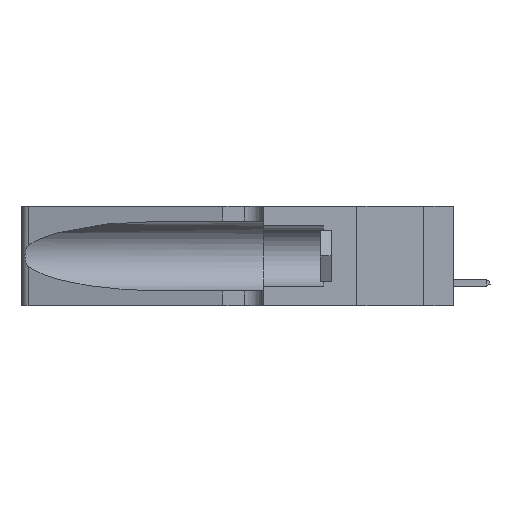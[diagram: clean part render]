
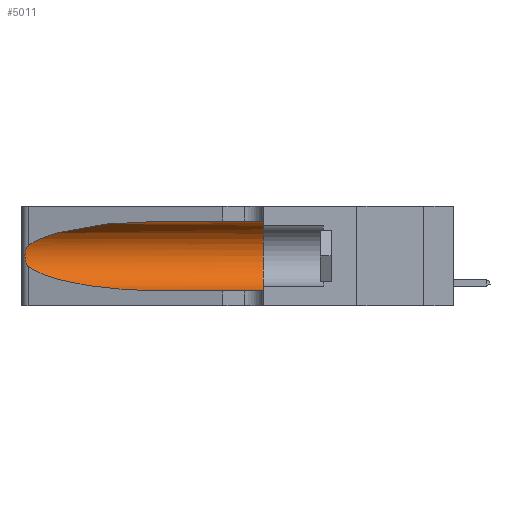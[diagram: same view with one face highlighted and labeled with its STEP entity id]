
A CAD part, left-side view. The second image highlights one B-rep face of the part: STEP entity #5011.
In plain terms, the highlighted cylindrical face has radius 3.308 mm (diameter 6.617 mm), a partial arc.
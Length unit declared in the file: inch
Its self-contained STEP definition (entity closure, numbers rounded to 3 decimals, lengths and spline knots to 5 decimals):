
#193 = EDGE_CURVE ( 'NONE', #3831, #10696, #7892, .T. ) ;
#352 = CARTESIAN_POINT ( 'NONE',  ( 0.1305, 0.35, 0.05475 ) ) ;
#851 = DIRECTION ( 'NONE',  ( 0., -1., 0. ) ) ;
#1454 = ORIENTED_EDGE ( 'NONE', *, *, #193, .T. ) ;
#1737 = CARTESIAN_POINT ( 'NONE',  ( 0.25854, 1.2359, 0.20912 ) ) ;
#1858 = CARTESIAN_POINT ( 'NONE',  ( 0.25487, 1.22718, 0.22369 ) ) ;
#1921 = CARTESIAN_POINT ( 'NONE',  ( 0.25789, 1.23486, 0.15765 ) ) ;
#2220 = CARTESIAN_POINT ( 'NONE',  ( 0.1305, 1.61858, 0.31525 ) ) ;
#2364 = EDGE_CURVE ( 'NONE', #7853, #3831, #17258, .T. ) ;
#3065 = ORIENTED_EDGE ( 'NONE', *, *, #10137, .T. ) ;
#3291 = CARTESIAN_POINT ( 'NONE',  ( 0.25639, 1.23186, 0.15144 ) ) ;
#3459 = LINE ( 'NONE', #2220, #13049 ) ;
#3567 = AXIS2_PLACEMENT_3D ( 'NONE', #7387, #4279, #14512 ) ;
#3663 = VECTOR ( 'NONE', #11412, 39.37008 ) ;
#3831 = VERTEX_POINT ( 'NONE', #13949 ) ;
#4229 = ORIENTED_EDGE ( 'NONE', *, *, #9082, .F. ) ;
#4279 = DIRECTION ( 'NONE',  ( 0., 1., 0. ) ) ;
#4333 = CYLINDRICAL_SURFACE ( 'NONE', #6088, 0.13025 ) ;
#4395 = CARTESIAN_POINT ( 'NONE',  ( 0.25555, 1.22994, 0.2215 ) ) ;
#4707 = CARTESIAN_POINT ( 'NONE',  ( 0.26017, 1.23833, 0.17102 ) ) ;
#4766 =( BOUNDED_CURVE ( )  B_SPLINE_CURVE ( 3, ( #9115, #17762, #9359, #6259 ),
 .UNSPECIFIED., .F., .T. ) 
 B_SPLINE_CURVE_WITH_KNOTS ( ( 4, 4 ),
 ( 1.5708, 2.84003 ),
 .UNSPECIFIED. ) 
 CURVE ( )  GEOMETRIC_REPRESENTATION_ITEM ( )  RATIONAL_B_SPLINE_CURVE ( ( 1., 0.87, 0.87, 1. ) ) 
 REPRESENTATION_ITEM ( '' )  );
#4895 = CARTESIAN_POINT ( 'NONE',  ( 0.25487, 1.22718, 0.14631 ) ) ;
#4959 = CARTESIAN_POINT ( 'NONE',  ( 0.26075, 1.23896, 0.19203 ) ) ;
#5011 = ADVANCED_FACE ( 'NONE', ( #8567 ), #4333, .F. ) ;
#5245 = VERTEX_POINT ( 'NONE', #8311 ) ;
#5905 = CARTESIAN_POINT ( 'NONE',  ( 0.25639, 1.23184, 0.21858 ) ) ;
#5938 = ORIENTED_EDGE ( 'NONE', *, *, #9003, .T. ) ;
#6088 = AXIS2_PLACEMENT_3D ( 'NONE', #13794, #12398, #15220 ) ;
#6259 = CARTESIAN_POINT ( 'NONE',  ( 0.25487, 1.22718, 0.22369 ) ) ;
#6638 = VERTEX_POINT ( 'NONE', #14657 ) ;
#7343 = CARTESIAN_POINT ( 'NONE',  ( 0.2373, 1.15595, 0.08982 ) ) ;
#7387 = CARTESIAN_POINT ( 'NONE',  ( 0.1305, 0.35, 0.185 ) ) ;
#7408 = CARTESIAN_POINT ( 'NONE',  ( 0.25487, 1.22718, 0.14631 ) ) ;
#7422 = CARTESIAN_POINT ( 'NONE',  ( 0.1305, 1.61858, 0.05475 ) ) ;
#7614 = CARTESIAN_POINT ( 'NONE',  ( 0.1305, 0.72297, 0.31525 ) ) ;
#7755 = CARTESIAN_POINT ( 'NONE',  ( 0.25555, 1.22993, 0.14849 ) ) ;
#7853 = VERTEX_POINT ( 'NONE', #14208 ) ;
#7892 = LINE ( 'NONE', #7422, #3663 ) ;
#8311 = CARTESIAN_POINT ( 'NONE',  ( 0.25487, 1.22718, 0.22369 ) ) ;
#8567 = FACE_OUTER_BOUND ( 'NONE', #14930, .T. ) ;
#9003 = EDGE_CURVE ( 'NONE', #16059, #5245, #4766, .T. ) ;
#9082 = EDGE_CURVE ( 'NONE', #6638, #10696, #15347, .T. ) ;
#9115 = CARTESIAN_POINT ( 'NONE',  ( 0.1305, 0.72297, 0.31525 ) ) ;
#9359 = CARTESIAN_POINT ( 'NONE',  ( 0.2373, 1.15595, 0.28018 ) ) ;
#10137 = EDGE_CURVE ( 'NONE', #5245, #7853, #15057, .T. ) ;
#10235 = CARTESIAN_POINT ( 'NONE',  ( 0.25787, 1.23484, 0.2124 ) ) ;
#10696 = VERTEX_POINT ( 'NONE', #352 ) ;
#11412 = DIRECTION ( 'NONE',  ( 0., -1., 0. ) ) ;
#11692 = CARTESIAN_POINT ( 'NONE',  ( 0.26018, 1.23835, 0.19895 ) ) ;
#11858 = EDGE_CURVE ( 'NONE', #16059, #6638, #3459, .T. ) ;
#11880 = CARTESIAN_POINT ( 'NONE',  ( 0.26075, 1.23896, 0.178 ) ) ;
#12398 = DIRECTION ( 'NONE',  ( 0., -1., 0. ) ) ;
#13049 = VECTOR ( 'NONE', #851, 39.37008 ) ;
#13094 = CARTESIAN_POINT ( 'NONE',  ( 0.1305, 0.72297, 0.05475 ) ) ;
#13436 = CARTESIAN_POINT ( 'NONE',  ( 0.25856, 1.23593, 0.16098 ) ) ;
#13794 = CARTESIAN_POINT ( 'NONE',  ( 0.1305, 1.61858, 0.185 ) ) ;
#13949 = CARTESIAN_POINT ( 'NONE',  ( 0.1305, 0.72297, 0.05475 ) ) ;
#14208 = CARTESIAN_POINT ( 'NONE',  ( 0.25487, 1.22718, 0.14631 ) ) ;
#14512 = DIRECTION ( 'NONE',  ( 0., 0., 1. ) ) ;
#14657 = CARTESIAN_POINT ( 'NONE',  ( 0.1305, 0.35, 0.31525 ) ) ;
#14930 = EDGE_LOOP ( 'NONE', ( #5938, #3065, #17496, #1454, #4229, #15394 ) ) ;
#15057 = B_SPLINE_CURVE_WITH_KNOTS ( 'NONE', 3,
 ( #1858, #4395, #5905, #10235, #1737, #11692, #4959, #11880, #4707, #13436, #1921, #3291, #7755, #4895 ),
 .UNSPECIFIED., .F., .F.,
 ( 4, 2, 2, 2, 2, 2, 4 ),
 ( 0., 0.00027, 0.00053, 0.00107, 0.0016, 0.00187, 0.00214 ),
 .UNSPECIFIED. ) ;
#15220 = DIRECTION ( 'NONE',  ( 0., 0., -1. ) ) ;
#15347 = CIRCLE ( 'NONE', #3567, 0.13025 ) ;
#15394 = ORIENTED_EDGE ( 'NONE', *, *, #11858, .F. ) ;
#16059 = VERTEX_POINT ( 'NONE', #7614 ) ;
#17258 =( BOUNDED_CURVE ( )  B_SPLINE_CURVE ( 3, ( #7408, #7343, #17356, #13094 ),
 .UNSPECIFIED., .F., .F. ) 
 B_SPLINE_CURVE_WITH_KNOTS ( ( 4, 4 ),
 ( 3.44316, 4.71239 ),
 .UNSPECIFIED. ) 
 CURVE ( )  GEOMETRIC_REPRESENTATION_ITEM ( )  RATIONAL_B_SPLINE_CURVE ( ( 1., 0.87, 0.87, 1. ) ) 
 REPRESENTATION_ITEM ( '' )  );
#17356 = CARTESIAN_POINT ( 'NONE',  ( 0.18966, 0.96281, 0.05475 ) ) ;
#17496 = ORIENTED_EDGE ( 'NONE', *, *, #2364, .T. ) ;
#17762 = CARTESIAN_POINT ( 'NONE',  ( 0.18966, 0.96281, 0.31525 ) ) ;
